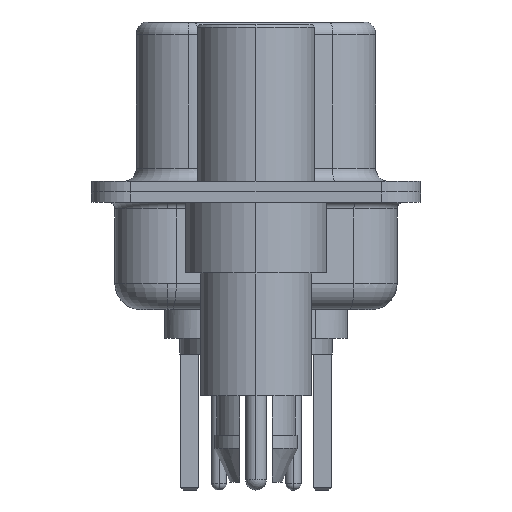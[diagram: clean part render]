
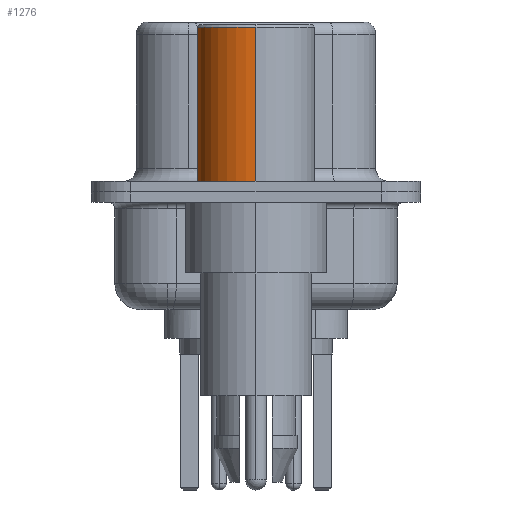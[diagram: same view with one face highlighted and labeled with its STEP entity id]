
A CAD part, left-side view. The second image highlights one B-rep face of the part: STEP entity #1276.
In plain terms, the highlighted cylindrical face has radius 2.25 mm (diameter 4.5 mm), a partial arc.
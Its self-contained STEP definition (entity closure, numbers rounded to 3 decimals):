
#214 = DIRECTION ( 'NONE',  ( 0., 0., 1. ) ) ;
#316 = AXIS2_PLACEMENT_3D ( 'NONE', #15245, #1724, #10659 ) ;
#584 = CARTESIAN_POINT ( 'NONE',  ( 0., 0., 0.4 ) ) ;
#996 = ORIENTED_EDGE ( 'NONE', *, *, #7001, .T. ) ;
#1276 = ADVANCED_FACE ( 'NONE', ( #3260 ), #7044, .T. ) ;
#1474 = VERTEX_POINT ( 'NONE', #10477 ) ;
#1724 = DIRECTION ( 'NONE',  ( 0., 0., 1. ) ) ;
#1790 = AXIS2_PLACEMENT_3D ( 'NONE', #584, #11944, #2243 ) ;
#1929 = VERTEX_POINT ( 'NONE', #10601 ) ;
#2178 = ORIENTED_EDGE ( 'NONE', *, *, #10361, .F. ) ;
#2243 = DIRECTION ( 'NONE',  ( 1., 0., 0. ) ) ;
#3205 = EDGE_CURVE ( 'NONE', #16619, #1474, #8992, .T. ) ;
#3260 = FACE_OUTER_BOUND ( 'NONE', #16439, .T. ) ;
#3743 = LINE ( 'NONE', #7293, #20743 ) ;
#4179 = CARTESIAN_POINT ( 'NONE',  ( -2.25, 0., 0.4 ) ) ;
#6322 = AXIS2_PLACEMENT_3D ( 'NONE', #8837, #20459, #10476 ) ;
#7001 = EDGE_CURVE ( 'NONE', #17543, #1929, #3743, .T. ) ;
#7044 = CYLINDRICAL_SURFACE ( 'NONE', #316, 2.25 ) ;
#7293 = CARTESIAN_POINT ( 'NONE',  ( -2.25, 0., 0.581 ) ) ;
#7978 = DIRECTION ( 'NONE',  ( 0., 0., 1. ) ) ;
#8235 = CARTESIAN_POINT ( 'NONE',  ( 2.25, 0., 0.581 ) ) ;
#8837 = CARTESIAN_POINT ( 'NONE',  ( 0., 0., 6.3 ) ) ;
#8992 = LINE ( 'NONE', #8235, #17337 ) ;
#10361 = EDGE_CURVE ( 'NONE', #1474, #1929, #18807, .T. ) ;
#10476 = DIRECTION ( 'NONE',  ( 1., 0., 0. ) ) ;
#10477 = CARTESIAN_POINT ( 'NONE',  ( 2.25, 0., 6.3 ) ) ;
#10601 = CARTESIAN_POINT ( 'NONE',  ( -2.25, 0., 6.3 ) ) ;
#10659 = DIRECTION ( 'NONE',  ( 1., 0., 0. ) ) ;
#10987 = CIRCLE ( 'NONE', #1790, 2.25 ) ;
#11944 = DIRECTION ( 'NONE',  ( 0., 0., 1. ) ) ;
#15245 = CARTESIAN_POINT ( 'NONE',  ( 0., 0., 0.581 ) ) ;
#16439 = EDGE_LOOP ( 'NONE', ( #21184, #996, #2178, #18443 ) ) ;
#16619 = VERTEX_POINT ( 'NONE', #18285 ) ;
#17337 = VECTOR ( 'NONE', #214, 1000. ) ;
#17543 = VERTEX_POINT ( 'NONE', #4179 ) ;
#18285 = CARTESIAN_POINT ( 'NONE',  ( 2.25, 0., 0.4 ) ) ;
#18443 = ORIENTED_EDGE ( 'NONE', *, *, #3205, .F. ) ;
#18807 = CIRCLE ( 'NONE', #6322, 2.25 ) ;
#20459 = DIRECTION ( 'NONE',  ( 0., 0., 1. ) ) ;
#20606 = EDGE_CURVE ( 'NONE', #16619, #17543, #10987, .T. ) ;
#20743 = VECTOR ( 'NONE', #7978, 1000. ) ;
#21184 = ORIENTED_EDGE ( 'NONE', *, *, #20606, .T. ) ;
